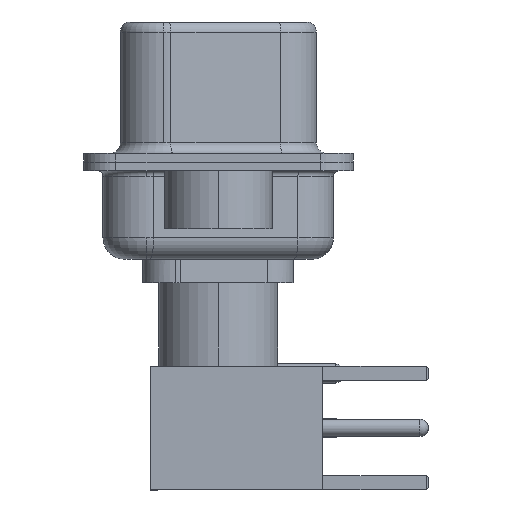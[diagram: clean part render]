
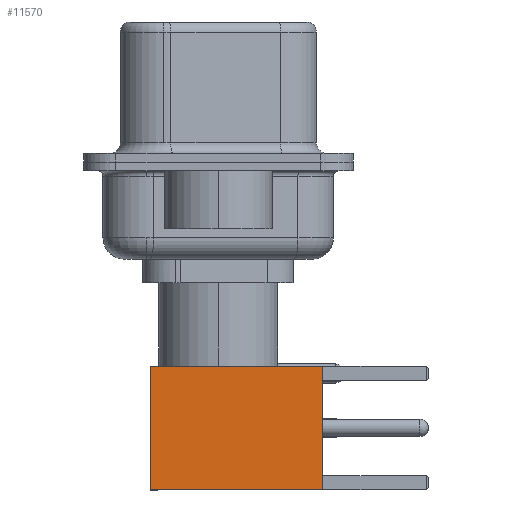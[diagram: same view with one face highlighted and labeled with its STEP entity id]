
A CAD part, left-side view. The second image highlights one B-rep face of the part: STEP entity #11570.
In plain terms, the highlighted face is planar.
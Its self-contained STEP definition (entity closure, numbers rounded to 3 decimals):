
#856 = PLANE ( 'NONE',  #8830 ) ;
#1258 = CARTESIAN_POINT ( 'NONE',  ( 0., 2.875, 8. ) ) ;
#1816 = EDGE_CURVE ( 'NONE', #28171, #25667, #4803, .T. ) ;
#3346 = CARTESIAN_POINT ( 'NONE',  ( -2.875, 2.875, 0. ) ) ;
#4614 = ORIENTED_EDGE ( 'NONE', *, *, #6030, .F. ) ;
#4803 = LINE ( 'NONE', #12269, #26143 ) ;
#5370 = DIRECTION ( 'NONE',  ( -1., 0., 0. ) ) ;
#5544 = EDGE_CURVE ( 'NONE', #13602, #28171, #20490, .T. ) ;
#5819 = EDGE_LOOP ( 'NONE', ( #12470, #21249, #4614, #26473 ) ) ;
#5850 = CARTESIAN_POINT ( 'NONE',  ( 2.875, 2.875, 0. ) ) ;
#6030 = EDGE_CURVE ( 'NONE', #12297, #25667, #7590, .T. ) ;
#6825 = CARTESIAN_POINT ( 'NONE',  ( -2.875, 2.875, 0. ) ) ;
#6997 = VECTOR ( 'NONE', #23417, 1000. ) ;
#7590 = LINE ( 'NONE', #3346, #21585 ) ;
#7603 = DIRECTION ( 'NONE',  ( 0., 1., 0. ) ) ;
#8025 = EDGE_CURVE ( 'NONE', #13602, #12297, #10236, .T. ) ;
#8830 = AXIS2_PLACEMENT_3D ( 'NONE', #5850, #7603, #14397 ) ;
#10062 = DIRECTION ( 'NONE',  ( -1., 0., 0. ) ) ;
#10236 = LINE ( 'NONE', #1258, #10628 ) ;
#10628 = VECTOR ( 'NONE', #5370, 1000. ) ;
#11074 = CARTESIAN_POINT ( 'NONE',  ( 2.875, 2.875, 0. ) ) ;
#11570 = ADVANCED_FACE ( 'NONE', ( #28325 ), #856, .T. ) ;
#12028 = DIRECTION ( 'NONE',  ( 0., 0., -1. ) ) ;
#12269 = CARTESIAN_POINT ( 'NONE',  ( 0., 2.875, 0. ) ) ;
#12297 = VERTEX_POINT ( 'NONE', #16951 ) ;
#12470 = ORIENTED_EDGE ( 'NONE', *, *, #5544, .T. ) ;
#13602 = VERTEX_POINT ( 'NONE', #19876 ) ;
#14397 = DIRECTION ( 'NONE',  ( 0., 0., 1. ) ) ;
#14459 = CARTESIAN_POINT ( 'NONE',  ( 2.875, 2.875, 0. ) ) ;
#16951 = CARTESIAN_POINT ( 'NONE',  ( -2.875, 2.875, 8. ) ) ;
#19876 = CARTESIAN_POINT ( 'NONE',  ( 2.875, 2.875, 8. ) ) ;
#20490 = LINE ( 'NONE', #14459, #6997 ) ;
#21249 = ORIENTED_EDGE ( 'NONE', *, *, #1816, .T. ) ;
#21585 = VECTOR ( 'NONE', #12028, 1000. ) ;
#23417 = DIRECTION ( 'NONE',  ( 0., 0., -1. ) ) ;
#25667 = VERTEX_POINT ( 'NONE', #6825 ) ;
#26143 = VECTOR ( 'NONE', #10062, 1000. ) ;
#26473 = ORIENTED_EDGE ( 'NONE', *, *, #8025, .F. ) ;
#28171 = VERTEX_POINT ( 'NONE', #11074 ) ;
#28325 = FACE_OUTER_BOUND ( 'NONE', #5819, .T. ) ;
